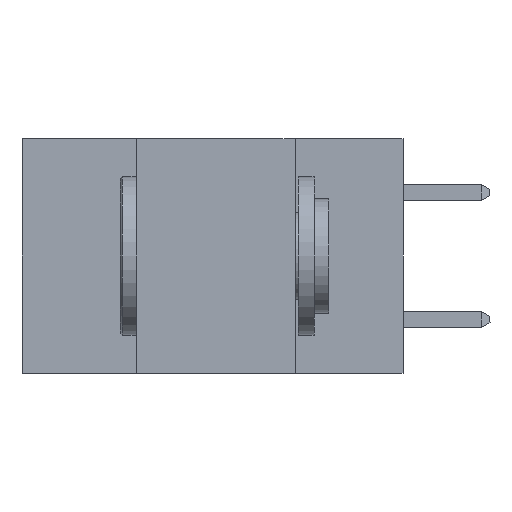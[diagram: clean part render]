
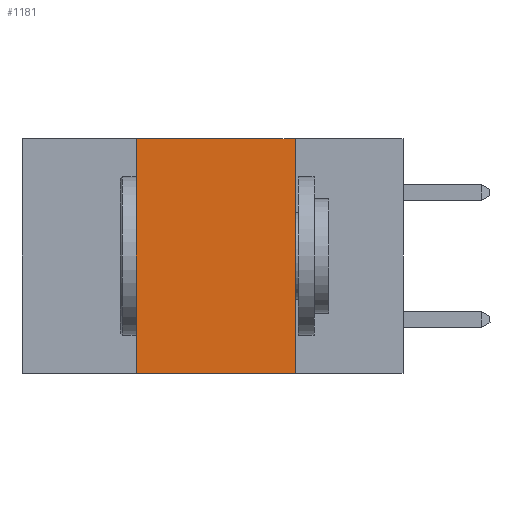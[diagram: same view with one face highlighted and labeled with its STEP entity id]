
A CAD part, left-side view. The second image highlights one B-rep face of the part: STEP entity #1181.
In plain terms, the highlighted planar face has unit normal (-1, 0, 0).
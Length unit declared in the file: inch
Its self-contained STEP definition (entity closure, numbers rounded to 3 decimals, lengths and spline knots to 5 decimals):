
#493 = VERTEX_POINT ( 'NONE', #974 ) ;
#974 = CARTESIAN_POINT ( 'NONE',  ( 0., 0.17, -0.37 ) ) ;
#1154 = DIRECTION ( 'NONE',  ( 0., 0., -1. ) ) ;
#1160 = DIRECTION ( 'NONE',  ( 1., 0., 0. ) ) ;
#1181 = ADVANCED_FACE ( 'NONE', ( #17224 ), #1539, .F. ) ;
#1539 = PLANE ( 'NONE',  #17902 ) ;
#1543 = CARTESIAN_POINT ( 'NONE',  ( 0., 0.17, 0. ) ) ;
#1849 = CARTESIAN_POINT ( 'NONE',  ( 0., 0.6, 0. ) ) ;
#1977 = VERTEX_POINT ( 'NONE', #17113 ) ;
#2582 = CARTESIAN_POINT ( 'NONE',  ( 0., 0.6, -0.37 ) ) ;
#4267 = VECTOR ( 'NONE', #6664, 39.37008 ) ;
#4543 = EDGE_LOOP ( 'NONE', ( #11900, #13291, #11549, #8121 ) ) ;
#6016 = VECTOR ( 'NONE', #17532, 39.37008 ) ;
#6664 = DIRECTION ( 'NONE',  ( 0., -1., 0. ) ) ;
#8121 = ORIENTED_EDGE ( 'NONE', *, *, #14820, .T. ) ;
#8220 = LINE ( 'NONE', #8315, #10956 ) ;
#8258 = LINE ( 'NONE', #13649, #11773 ) ;
#8315 = CARTESIAN_POINT ( 'NONE',  ( 0., 0.17, 0. ) ) ;
#8813 = LINE ( 'NONE', #12666, #4267 ) ;
#9325 = CARTESIAN_POINT ( 'NONE',  ( 0., 0.42, 0. ) ) ;
#9529 = VERTEX_POINT ( 'NONE', #1543 ) ;
#9823 = DIRECTION ( 'NONE',  ( 0., 0., -1. ) ) ;
#10043 = LINE ( 'NONE', #2582, #6016 ) ;
#10938 = EDGE_CURVE ( 'NONE', #15118, #9529, #8813, .T. ) ;
#10956 = VECTOR ( 'NONE', #9823, 39.37008 ) ;
#11549 = ORIENTED_EDGE ( 'NONE', *, *, #18838, .F. ) ;
#11773 = VECTOR ( 'NONE', #15132, 39.37008 ) ;
#11900 = ORIENTED_EDGE ( 'NONE', *, *, #14020, .F. ) ;
#12666 = CARTESIAN_POINT ( 'NONE',  ( 0., 0.6, 0. ) ) ;
#13291 = ORIENTED_EDGE ( 'NONE', *, *, #10938, .F. ) ;
#13649 = CARTESIAN_POINT ( 'NONE',  ( 0., 0.42, 0. ) ) ;
#14020 = EDGE_CURVE ( 'NONE', #9529, #493, #8220, .T. ) ;
#14820 = EDGE_CURVE ( 'NONE', #1977, #493, #10043, .T. ) ;
#15118 = VERTEX_POINT ( 'NONE', #9325 ) ;
#15132 = DIRECTION ( 'NONE',  ( 0., 0., 1. ) ) ;
#17113 = CARTESIAN_POINT ( 'NONE',  ( 0., 0.42, -0.37 ) ) ;
#17224 = FACE_OUTER_BOUND ( 'NONE', #4543, .T. ) ;
#17532 = DIRECTION ( 'NONE',  ( 0., -1., 0. ) ) ;
#17902 = AXIS2_PLACEMENT_3D ( 'NONE', #1849, #1160, #1154 ) ;
#18838 = EDGE_CURVE ( 'NONE', #1977, #15118, #8258, .T. ) ;
